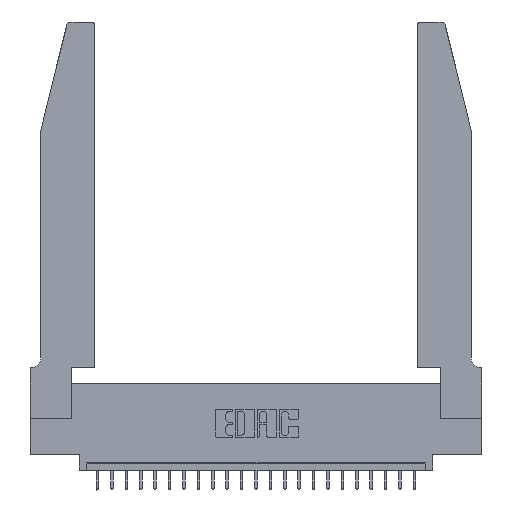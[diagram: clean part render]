
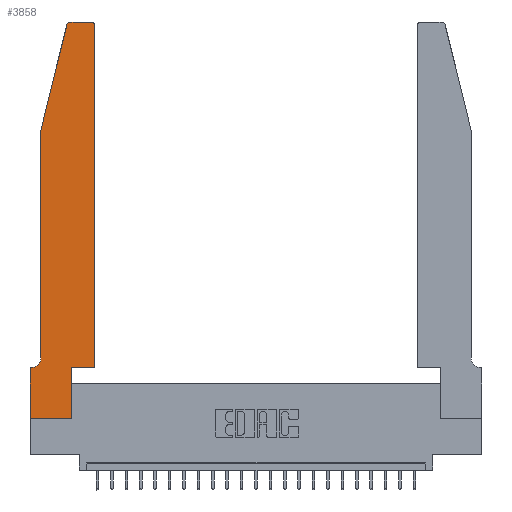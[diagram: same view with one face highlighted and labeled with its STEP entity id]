
A CAD part, top view. The second image highlights one B-rep face of the part: STEP entity #3858.
In plain terms, the highlighted planar face has unit normal (0, 0, 1).
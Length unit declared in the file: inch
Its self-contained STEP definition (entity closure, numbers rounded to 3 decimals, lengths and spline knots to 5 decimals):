
#190 = VERTEX_POINT ( 'NONE', #5678 ) ;
#564 = CARTESIAN_POINT ( 'NONE',  ( 0.2865, 0.35, 0.37 ) ) ;
#677 = DIRECTION ( 'NONE',  ( 1., 0., 0. ) ) ;
#714 = CARTESIAN_POINT ( 'NONE',  ( 0.4505, 0.35, 0.37 ) ) ;
#812 = CARTESIAN_POINT ( 'NONE',  ( 0.4505, 2.72, 0.37 ) ) ;
#1037 = PLANE ( 'NONE',  #1734 ) ;
#1264 = DIRECTION ( 'NONE',  ( -0.239, -0.971, 0. ) ) ;
#1268 = DIRECTION ( 'NONE',  ( 0., -1., 0. ) ) ;
#1684 = VECTOR ( 'NONE', #20124, 39.37008 ) ;
#1734 = AXIS2_PLACEMENT_3D ( 'NONE', #16018, #17908, #22175 ) ;
#2013 = DIRECTION ( 'NONE',  ( -1., 0., 0. ) ) ;
#2499 = EDGE_CURVE ( 'NONE', #2946, #4559, #4653, .T. ) ;
#2515 = EDGE_CURVE ( 'NONE', #10561, #12742, #12331, .T. ) ;
#2712 = CARTESIAN_POINT ( 'NONE',  ( 0.2865, 0., 0.37 ) ) ;
#2735 = DIRECTION ( 'NONE',  ( 1., 0., 0. ) ) ;
#2764 = ORIENTED_EDGE ( 'NONE', *, *, #23985, .T. ) ;
#2946 = VERTEX_POINT ( 'NONE', #714 ) ;
#3078 = ORIENTED_EDGE ( 'NONE', *, *, #22442, .T. ) ;
#3422 = CARTESIAN_POINT ( 'NONE',  ( 0.0055, 0.42, 0.37 ) ) ;
#3491 = VERTEX_POINT ( 'NONE', #10873 ) ;
#3552 = CARTESIAN_POINT ( 'NONE',  ( 0.0055, 0.35, 0.37 ) ) ;
#3858 = ADVANCED_FACE ( 'NONE', ( #10224 ), #1037, .T. ) ;
#4449 = DIRECTION ( 'NONE',  ( 0., 0., 1. ) ) ;
#4559 = VERTEX_POINT ( 'NONE', #812 ) ;
#4653 = LINE ( 'NONE', #18363, #1684 ) ;
#4698 = CARTESIAN_POINT ( 'NONE',  ( 0.4205, 2.72, 0.37 ) ) ;
#5012 = CARTESIAN_POINT ( 'NONE',  ( 0.0755, 0.42, 0.37 ) ) ;
#5381 = CARTESIAN_POINT ( 'NONE',  ( 0.284, 2.75, 0.37 ) ) ;
#5434 = DIRECTION ( 'NONE',  ( -1., 0., 0. ) ) ;
#5678 = CARTESIAN_POINT ( 'NONE',  ( 0.25487, 2.72718, 0.37 ) ) ;
#5749 = ORIENTED_EDGE ( 'NONE', *, *, #20394, .T. ) ;
#5811 = ORIENTED_EDGE ( 'NONE', *, *, #14825, .T. ) ;
#7472 = ORIENTED_EDGE ( 'NONE', *, *, #20896, .T. ) ;
#7550 = VECTOR ( 'NONE', #2735, 39.37008 ) ;
#7563 = DIRECTION ( 'NONE',  ( 0., 0., -1. ) ) ;
#7571 = VERTEX_POINT ( 'NONE', #9665 ) ;
#8066 = VECTOR ( 'NONE', #13284, 39.37008 ) ;
#8516 = VECTOR ( 'NONE', #24015, 39.37008 ) ;
#8832 = VECTOR ( 'NONE', #2013, 39.37008 ) ;
#9381 = LINE ( 'NONE', #13992, #8066 ) ;
#9431 = ORIENTED_EDGE ( 'NONE', *, *, #15790, .T. ) ;
#9665 = CARTESIAN_POINT ( 'NONE',  ( 0., 0., 0.37 ) ) ;
#9961 = EDGE_CURVE ( 'NONE', #17421, #2946, #13958, .T. ) ;
#10004 = VERTEX_POINT ( 'NONE', #5012 ) ;
#10105 = AXIS2_PLACEMENT_3D ( 'NONE', #11897, #19563, #677 ) ;
#10224 = FACE_OUTER_BOUND ( 'NONE', #24604, .T. ) ;
#10561 = VERTEX_POINT ( 'NONE', #3552 ) ;
#10577 = LINE ( 'NONE', #20403, #18865 ) ;
#10873 = CARTESIAN_POINT ( 'NONE',  ( 0.4205, 2.75, 0.37 ) ) ;
#11246 = ORIENTED_EDGE ( 'NONE', *, *, #12398, .T. ) ;
#11336 = CARTESIAN_POINT ( 'NONE',  ( 0.0755, 2., 0.37 ) ) ;
#11849 = AXIS2_PLACEMENT_3D ( 'NONE', #4698, #4449, #12263 ) ;
#11897 = CARTESIAN_POINT ( 'NONE',  ( 0.284, 2.72, 0.37 ) ) ;
#12263 = DIRECTION ( 'NONE',  ( 1., 0., 0. ) ) ;
#12331 = LINE ( 'NONE', #22003, #8516 ) ;
#12398 = EDGE_CURVE ( 'NONE', #7571, #21788, #14079, .T. ) ;
#12742 = VERTEX_POINT ( 'NONE', #23856 ) ;
#13284 = DIRECTION ( 'NONE',  ( 0., 1., 0. ) ) ;
#13617 = VECTOR ( 'NONE', #17767, 39.37008 ) ;
#13838 = CARTESIAN_POINT ( 'NONE',  ( 0.4505, 0.35, 0.37 ) ) ;
#13958 = LINE ( 'NONE', #13838, #7550 ) ;
#13992 = CARTESIAN_POINT ( 'NONE',  ( 0.2865, 0.35, 0.37 ) ) ;
#14003 = VERTEX_POINT ( 'NONE', #5381 ) ;
#14079 = LINE ( 'NONE', #17859, #17287 ) ;
#14481 = LINE ( 'NONE', #18502, #22932 ) ;
#14553 = EDGE_CURVE ( 'NONE', #21788, #17421, #9381, .T. ) ;
#14825 = EDGE_CURVE ( 'NONE', #190, #21686, #14481, .T. ) ;
#15243 = LINE ( 'NONE', #19008, #8832 ) ;
#15790 = EDGE_CURVE ( 'NONE', #14003, #190, #23759, .T. ) ;
#15865 = CIRCLE ( 'NONE', #21078, 0.07 ) ;
#15995 = ORIENTED_EDGE ( 'NONE', *, *, #2515, .T. ) ;
#16018 = CARTESIAN_POINT ( 'NONE',  ( 0., 0.35, 0.37 ) ) ;
#16089 = DIRECTION ( 'NONE',  ( 1., 0., 0. ) ) ;
#16420 = ORIENTED_EDGE ( 'NONE', *, *, #9961, .T. ) ;
#17287 = VECTOR ( 'NONE', #16089, 39.37008 ) ;
#17421 = VERTEX_POINT ( 'NONE', #564 ) ;
#17749 = ORIENTED_EDGE ( 'NONE', *, *, #23827, .T. ) ;
#17767 = DIRECTION ( 'NONE',  ( 0., -1., 0. ) ) ;
#17859 = CARTESIAN_POINT ( 'NONE',  ( 0., 0., 0.37 ) ) ;
#17908 = DIRECTION ( 'NONE',  ( 0., 0., 1. ) ) ;
#18363 = CARTESIAN_POINT ( 'NONE',  ( 0.4505, 0.35, 0.37 ) ) ;
#18502 = CARTESIAN_POINT ( 'NONE',  ( 0.0755, 2., 0.37 ) ) ;
#18865 = VECTOR ( 'NONE', #1268, 39.37008 ) ;
#19008 = CARTESIAN_POINT ( 'NONE',  ( 0.2605, 2.75, 0.37 ) ) ;
#19082 = CIRCLE ( 'NONE', #11849, 0.03 ) ;
#19563 = DIRECTION ( 'NONE',  ( 0., 0., 1. ) ) ;
#20021 = LINE ( 'NONE', #21779, #13617 ) ;
#20124 = DIRECTION ( 'NONE',  ( 0., 1., 0. ) ) ;
#20394 = EDGE_CURVE ( 'NONE', #10004, #10561, #15865, .T. ) ;
#20403 = CARTESIAN_POINT ( 'NONE',  ( 0.0755, 2., 0.37 ) ) ;
#20896 = EDGE_CURVE ( 'NONE', #4559, #3491, #19082, .T. ) ;
#21078 = AXIS2_PLACEMENT_3D ( 'NONE', #3422, #7563, #5434 ) ;
#21686 = VERTEX_POINT ( 'NONE', #11336 ) ;
#21779 = CARTESIAN_POINT ( 'NONE',  ( 0., 0., 0.37 ) ) ;
#21788 = VERTEX_POINT ( 'NONE', #2712 ) ;
#22003 = CARTESIAN_POINT ( 'NONE',  ( 0.0755, 0.35, 0.37 ) ) ;
#22175 = DIRECTION ( 'NONE',  ( 1., 0., 0. ) ) ;
#22306 = ORIENTED_EDGE ( 'NONE', *, *, #2499, .T. ) ;
#22442 = EDGE_CURVE ( 'NONE', #12742, #7571, #20021, .T. ) ;
#22932 = VECTOR ( 'NONE', #1264, 39.37008 ) ;
#23218 = ORIENTED_EDGE ( 'NONE', *, *, #14553, .T. ) ;
#23759 = CIRCLE ( 'NONE', #10105, 0.03 ) ;
#23827 = EDGE_CURVE ( 'NONE', #21686, #10004, #10577, .T. ) ;
#23856 = CARTESIAN_POINT ( 'NONE',  ( 0., 0.35, 0.37 ) ) ;
#23985 = EDGE_CURVE ( 'NONE', #3491, #14003, #15243, .T. ) ;
#24015 = DIRECTION ( 'NONE',  ( -1., 0., 0. ) ) ;
#24604 = EDGE_LOOP ( 'NONE', ( #2764, #9431, #5811, #17749, #5749, #15995, #3078, #11246, #23218, #16420, #22306, #7472 ) ) ;
